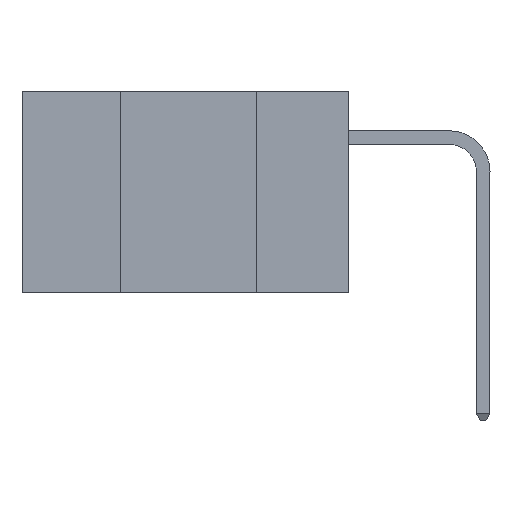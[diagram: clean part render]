
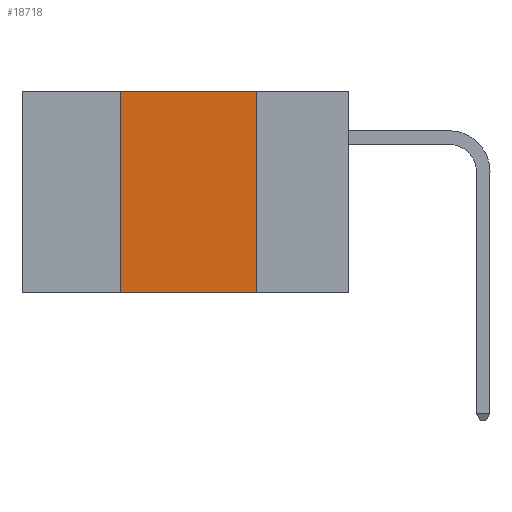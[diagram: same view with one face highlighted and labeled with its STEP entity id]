
A CAD part, left-side view. The second image highlights one B-rep face of the part: STEP entity #18718.
In plain terms, the highlighted planar face has unit normal (-1, 0, 0).
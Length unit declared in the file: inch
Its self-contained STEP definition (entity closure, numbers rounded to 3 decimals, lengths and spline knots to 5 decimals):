
#341 = VERTEX_POINT ( 'NONE', #6801 ) ;
#1080 = EDGE_CURVE ( 'NONE', #10983, #12430, #8240, .T. ) ;
#2933 = DIRECTION ( 'NONE',  ( 0., -1., 0. ) ) ;
#2995 = ORIENTED_EDGE ( 'NONE', *, *, #8283, .T. ) ;
#3296 = CARTESIAN_POINT ( 'NONE',  ( 0., 0.6, 0. ) ) ;
#3789 = VECTOR ( 'NONE', #16504, 39.37008 ) ;
#4892 = DIRECTION ( 'NONE',  ( 1., 0., 0. ) ) ;
#5218 = LINE ( 'NONE', #6706, #14326 ) ;
#5435 = CARTESIAN_POINT ( 'NONE',  ( 0., 0.17, -0.37 ) ) ;
#6706 = CARTESIAN_POINT ( 'NONE',  ( 0., 0.42, 0. ) ) ;
#6801 = CARTESIAN_POINT ( 'NONE',  ( 0., 0.42, 0. ) ) ;
#7402 = ORIENTED_EDGE ( 'NONE', *, *, #16846, .F. ) ;
#7626 = ORIENTED_EDGE ( 'NONE', *, *, #13813, .F. ) ;
#7756 = VECTOR ( 'NONE', #10985, 39.37008 ) ;
#8108 = EDGE_LOOP ( 'NONE', ( #9074, #7402, #7626, #2995 ) ) ;
#8219 = FACE_OUTER_BOUND ( 'NONE', #8108, .T. ) ;
#8240 = LINE ( 'NONE', #15641, #7756 ) ;
#8283 = EDGE_CURVE ( 'NONE', #16401, #12430, #16066, .T. ) ;
#8317 = DIRECTION ( 'NONE',  ( 0., 0., 1. ) ) ;
#9074 = ORIENTED_EDGE ( 'NONE', *, *, #1080, .F. ) ;
#9081 = CARTESIAN_POINT ( 'NONE',  ( 0., 0.6, 0. ) ) ;
#9624 = VECTOR ( 'NONE', #2933, 39.37008 ) ;
#10983 = VERTEX_POINT ( 'NONE', #18649 ) ;
#10985 = DIRECTION ( 'NONE',  ( 0., 0., -1. ) ) ;
#12430 = VERTEX_POINT ( 'NONE', #5435 ) ;
#12520 = PLANE ( 'NONE',  #15401 ) ;
#13472 = CARTESIAN_POINT ( 'NONE',  ( 0., 0.6, -0.37 ) ) ;
#13743 = LINE ( 'NONE', #9081, #9624 ) ;
#13813 = EDGE_CURVE ( 'NONE', #16401, #341, #5218, .T. ) ;
#14326 = VECTOR ( 'NONE', #8317, 39.37008 ) ;
#15401 = AXIS2_PLACEMENT_3D ( 'NONE', #3296, #4892, #15607 ) ;
#15607 = DIRECTION ( 'NONE',  ( 0., 0., -1. ) ) ;
#15641 = CARTESIAN_POINT ( 'NONE',  ( 0., 0.17, 0. ) ) ;
#16066 = LINE ( 'NONE', #13472, #3789 ) ;
#16401 = VERTEX_POINT ( 'NONE', #18888 ) ;
#16504 = DIRECTION ( 'NONE',  ( 0., -1., 0. ) ) ;
#16846 = EDGE_CURVE ( 'NONE', #341, #10983, #13743, .T. ) ;
#18649 = CARTESIAN_POINT ( 'NONE',  ( 0., 0.17, 0. ) ) ;
#18718 = ADVANCED_FACE ( 'NONE', ( #8219 ), #12520, .F. ) ;
#18888 = CARTESIAN_POINT ( 'NONE',  ( 0., 0.42, -0.37 ) ) ;
